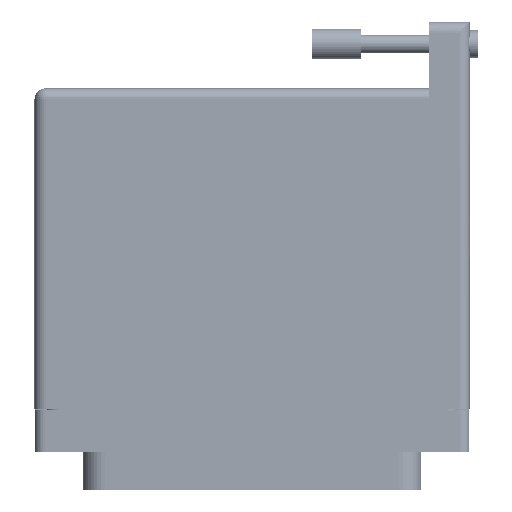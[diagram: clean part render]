
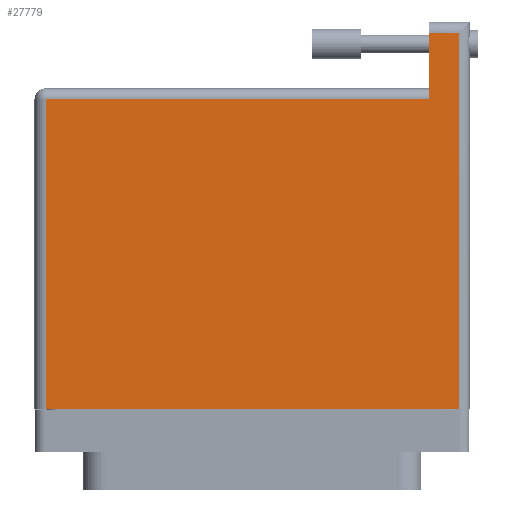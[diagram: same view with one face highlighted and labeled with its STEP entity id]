
A CAD part, front view. The second image highlights one B-rep face of the part: STEP entity #27779.
In plain terms, the highlighted face is planar.
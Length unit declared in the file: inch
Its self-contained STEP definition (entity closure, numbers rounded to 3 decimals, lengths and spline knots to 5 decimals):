
#1192 = VERTEX_POINT ( 'NONE', #68085 ) ;
#7741 = ORIENTED_EDGE ( 'NONE', *, *, #76139, .T. ) ;
#9399 = ORIENTED_EDGE ( 'NONE', *, *, #48159, .T. ) ;
#11772 = EDGE_CURVE ( 'NONE', #52931, #80096, #77553, .T. ) ;
#12685 = CARTESIAN_POINT ( 'NONE',  ( 1.1215, 1.86, 0.765 ) ) ;
#13789 = LINE ( 'NONE', #84174, #40404 ) ;
#15908 = DIRECTION ( 'NONE',  ( 0., -1., 0. ) ) ;
#16262 = DIRECTION ( 'NONE',  ( 0., -1., 0. ) ) ;
#17665 = VERTEX_POINT ( 'NONE', #76712 ) ;
#18902 = CARTESIAN_POINT ( 'NONE',  ( -1.3075, 1.86, 0.765 ) ) ;
#20147 = DIRECTION ( 'NONE',  ( 0., 1., 0. ) ) ;
#20958 = VECTOR ( 'NONE', #16262, 39.37008 ) ;
#22338 = PLANE ( 'NONE',  #52330 ) ;
#26505 = VERTEX_POINT ( 'NONE', #79104 ) ;
#27196 = LINE ( 'NONE', #55803, #74209 ) ;
#27779 = ADVANCED_FACE ( 'NONE', ( #92727 ), #22338, .F. ) ;
#27820 = DIRECTION ( 'NONE',  ( -1., 0., 0. ) ) ;
#28245 = EDGE_CURVE ( 'NONE', #1192, #26505, #13789, .T. ) ;
#28991 = VERTEX_POINT ( 'NONE', #83844 ) ;
#29439 = CARTESIAN_POINT ( 'NONE',  ( -1.3775, 2.28, 0.765 ) ) ;
#32691 = ORIENTED_EDGE ( 'NONE', *, *, #89853, .T. ) ;
#34446 = DIRECTION ( 'NONE',  ( 1., 0., 0. ) ) ;
#37830 = LINE ( 'NONE', #73039, #20958 ) ;
#38992 = EDGE_LOOP ( 'NONE', ( #7741, #89443, #9399, #69208, #32691, #42626 ) ) ;
#40404 = VECTOR ( 'NONE', #34446, 39.37008 ) ;
#41953 = EDGE_CURVE ( 'NONE', #28991, #17665, #79173, .T. ) ;
#42626 = ORIENTED_EDGE ( 'NONE', *, *, #41953, .T. ) ;
#48159 = EDGE_CURVE ( 'NONE', #80096, #1192, #37830, .T. ) ;
#49102 = DIRECTION ( 'NONE',  ( -1., 0., 0. ) ) ;
#49567 = CARTESIAN_POINT ( 'NONE',  ( -1.3775, 1.93, 0.765 ) ) ;
#51715 = VECTOR ( 'NONE', #27820, 39.37008 ) ;
#52330 = AXIS2_PLACEMENT_3D ( 'NONE', #49567, #79568, #49102 ) ;
#52931 = VERTEX_POINT ( 'NONE', #12685 ) ;
#55803 = CARTESIAN_POINT ( 'NONE',  ( 1.3075, 2.35, 0.765 ) ) ;
#57586 = DIRECTION ( 'NONE',  ( -1., 0., 0. ) ) ;
#57748 = VECTOR ( 'NONE', #57586, 39.37008 ) ;
#59932 = VECTOR ( 'NONE', #15908, 39.37008 ) ;
#67038 = LINE ( 'NONE', #81101, #59932 ) ;
#68085 = CARTESIAN_POINT ( 'NONE',  ( -1.3075, -0.1, 0.765 ) ) ;
#69208 = ORIENTED_EDGE ( 'NONE', *, *, #28245, .T. ) ;
#70034 = CARTESIAN_POINT ( 'NONE',  ( -1.3775, 1.86, 0.765 ) ) ;
#73039 = CARTESIAN_POINT ( 'NONE',  ( -1.3075, -0.1, 0.765 ) ) ;
#74209 = VECTOR ( 'NONE', #20147, 39.37008 ) ;
#76139 = EDGE_CURVE ( 'NONE', #17665, #52931, #67038, .T. ) ;
#76712 = CARTESIAN_POINT ( 'NONE',  ( 1.1215, 2.28, 0.765 ) ) ;
#77553 = LINE ( 'NONE', #70034, #51715 ) ;
#79104 = CARTESIAN_POINT ( 'NONE',  ( 1.3075, -0.1, 0.765 ) ) ;
#79173 = LINE ( 'NONE', #29439, #57748 ) ;
#79568 = DIRECTION ( 'NONE',  ( 0., 0., -1. ) ) ;
#80096 = VERTEX_POINT ( 'NONE', #18902 ) ;
#81101 = CARTESIAN_POINT ( 'NONE',  ( 1.1215, 2.35, 0.765 ) ) ;
#83844 = CARTESIAN_POINT ( 'NONE',  ( 1.3075, 2.28, 0.765 ) ) ;
#84174 = CARTESIAN_POINT ( 'NONE',  ( -1.3775, -0.1, 0.765 ) ) ;
#89443 = ORIENTED_EDGE ( 'NONE', *, *, #11772, .T. ) ;
#89853 = EDGE_CURVE ( 'NONE', #26505, #28991, #27196, .T. ) ;
#92727 = FACE_OUTER_BOUND ( 'NONE', #38992, .T. ) ;
